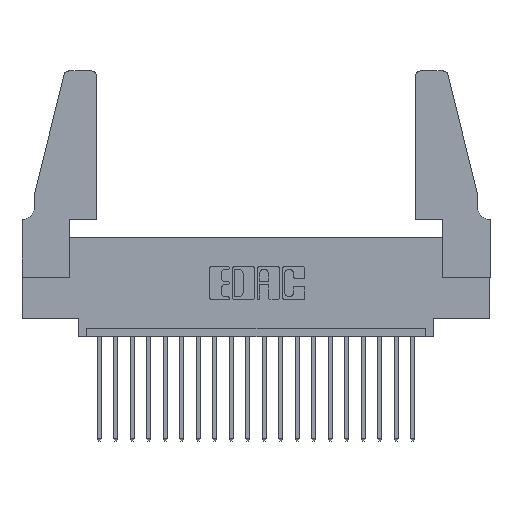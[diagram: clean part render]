
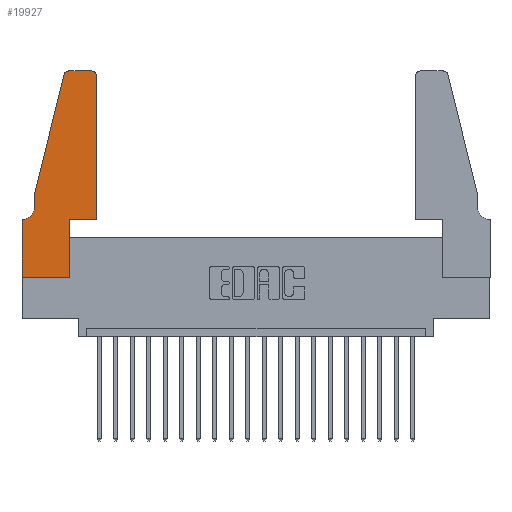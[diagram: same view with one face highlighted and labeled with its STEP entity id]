
A CAD part, top view. The second image highlights one B-rep face of the part: STEP entity #19927.
In plain terms, the highlighted planar face has unit normal (0, 0, 1).
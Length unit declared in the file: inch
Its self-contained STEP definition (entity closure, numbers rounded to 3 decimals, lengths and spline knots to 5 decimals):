
#42 = ORIENTED_EDGE ( 'NONE', *, *, #7718, .T. ) ;
#100 = EDGE_CURVE ( 'NONE', #8436, #19160, #12541, .T. ) ;
#278 = DIRECTION ( 'NONE',  ( 1., 0., 0. ) ) ;
#500 = DIRECTION ( 'NONE',  ( 1., 0., 0. ) ) ;
#636 = DIRECTION ( 'NONE',  ( 0., -1., 0. ) ) ;
#661 = CARTESIAN_POINT ( 'NONE',  ( 0.0755, 0.35, 0.37 ) ) ;
#727 = AXIS2_PLACEMENT_3D ( 'NONE', #11639, #16395, #500 ) ;
#766 = DIRECTION ( 'NONE',  ( -0.239, -0.971, 0. ) ) ;
#945 = DIRECTION ( 'NONE',  ( 0., 0., 1. ) ) ;
#1049 = DIRECTION ( 'NONE',  ( -1., 0., 0. ) ) ;
#1065 = CARTESIAN_POINT ( 'NONE',  ( 0.284, 1.25, 0.37 ) ) ;
#1090 = LINE ( 'NONE', #8948, #9182 ) ;
#1420 = CARTESIAN_POINT ( 'NONE',  ( 0., 0., 0.37 ) ) ;
#1441 = CARTESIAN_POINT ( 'NONE',  ( 0.0755, 0.5, 0.37 ) ) ;
#1651 = VERTEX_POINT ( 'NONE', #19047 ) ;
#1655 = EDGE_CURVE ( 'NONE', #8353, #12202, #19097, .T. ) ;
#1698 = FACE_OUTER_BOUND ( 'NONE', #18260, .T. ) ;
#2104 = VERTEX_POINT ( 'NONE', #13752 ) ;
#2261 = ORIENTED_EDGE ( 'NONE', *, *, #10839, .T. ) ;
#2407 = CARTESIAN_POINT ( 'NONE',  ( 0.4505, 1.22, 0.37 ) ) ;
#2546 = VERTEX_POINT ( 'NONE', #13347 ) ;
#2612 = ORIENTED_EDGE ( 'NONE', *, *, #1655, .T. ) ;
#3149 = CARTESIAN_POINT ( 'NONE',  ( 0., 0.35, 0.37 ) ) ;
#3569 = ORIENTED_EDGE ( 'NONE', *, *, #5462, .T. ) ;
#3583 = VECTOR ( 'NONE', #766, 39.37008 ) ;
#3682 = CARTESIAN_POINT ( 'NONE',  ( 0.0055, 0.35, 0.37 ) ) ;
#3754 = VERTEX_POINT ( 'NONE', #14159 ) ;
#3808 = EDGE_CURVE ( 'NONE', #2104, #8353, #8250, .T. ) ;
#3920 = VECTOR ( 'NONE', #636, 39.37008 ) ;
#4205 = CIRCLE ( 'NONE', #6808, 0.07 ) ;
#4263 = VERTEX_POINT ( 'NONE', #3682 ) ;
#4315 = DIRECTION ( 'NONE',  ( -1., 0., 0. ) ) ;
#4437 = CARTESIAN_POINT ( 'NONE',  ( 0.4505, 0.35, 0.37 ) ) ;
#4447 = DIRECTION ( 'NONE',  ( 1., 0., 0. ) ) ;
#5462 = EDGE_CURVE ( 'NONE', #19718, #19481, #8505, .T. ) ;
#6401 = LINE ( 'NONE', #661, #8649 ) ;
#6675 = CARTESIAN_POINT ( 'NONE',  ( 0., 0., 0.37 ) ) ;
#6808 = AXIS2_PLACEMENT_3D ( 'NONE', #20013, #18310, #15224 ) ;
#6945 = CARTESIAN_POINT ( 'NONE',  ( 0.0755, 0.5, 0.37 ) ) ;
#6960 = EDGE_CURVE ( 'NONE', #19160, #2546, #8687, .T. ) ;
#7383 = CARTESIAN_POINT ( 'NONE',  ( 0.4205, 1.22, 0.37 ) ) ;
#7718 = EDGE_CURVE ( 'NONE', #4263, #8436, #6401, .T. ) ;
#7729 = VERTEX_POINT ( 'NONE', #1065 ) ;
#8171 = ORIENTED_EDGE ( 'NONE', *, *, #6960, .T. ) ;
#8250 = LINE ( 'NONE', #4437, #19176 ) ;
#8353 = VERTEX_POINT ( 'NONE', #15241 ) ;
#8436 = VERTEX_POINT ( 'NONE', #15012 ) ;
#8505 = LINE ( 'NONE', #12013, #3583 ) ;
#8596 = ORIENTED_EDGE ( 'NONE', *, *, #10520, .T. ) ;
#8649 = VECTOR ( 'NONE', #4315, 39.37008 ) ;
#8687 = LINE ( 'NONE', #6675, #15054 ) ;
#8767 = ORIENTED_EDGE ( 'NONE', *, *, #19090, .T. ) ;
#8900 = ORIENTED_EDGE ( 'NONE', *, *, #3808, .T. ) ;
#8948 = CARTESIAN_POINT ( 'NONE',  ( 0.2605, 1.25, 0.37 ) ) ;
#8990 = DIRECTION ( 'NONE',  ( 1., 0., 0. ) ) ;
#9182 = VECTOR ( 'NONE', #1049, 39.37008 ) ;
#9311 = LINE ( 'NONE', #11354, #17394 ) ;
#9631 = EDGE_CURVE ( 'NONE', #19481, #3754, #16663, .T. ) ;
#9711 = DIRECTION ( 'NONE',  ( 0., 1., 0. ) ) ;
#9851 = CARTESIAN_POINT ( 'NONE',  ( 0.4505, 0.35, 0.37 ) ) ;
#10071 = EDGE_CURVE ( 'NONE', #12202, #1651, #16834, .T. ) ;
#10520 = EDGE_CURVE ( 'NONE', #1651, #7729, #1090, .T. ) ;
#10839 = EDGE_CURVE ( 'NONE', #7729, #19718, #11644, .T. ) ;
#11354 = CARTESIAN_POINT ( 'NONE',  ( 0.2865, 0.35, 0.37 ) ) ;
#11639 = CARTESIAN_POINT ( 'NONE',  ( 0.284, 1.22, 0.37 ) ) ;
#11644 = CIRCLE ( 'NONE', #727, 0.03 ) ;
#12013 = CARTESIAN_POINT ( 'NONE',  ( 0.0755, 0.5, 0.37 ) ) ;
#12202 = VERTEX_POINT ( 'NONE', #2407 ) ;
#12541 = LINE ( 'NONE', #1420, #17707 ) ;
#13213 = ORIENTED_EDGE ( 'NONE', *, *, #9631, .T. ) ;
#13347 = CARTESIAN_POINT ( 'NONE',  ( 0.2865, 0., 0.37 ) ) ;
#13750 = ORIENTED_EDGE ( 'NONE', *, *, #18132, .T. ) ;
#13752 = CARTESIAN_POINT ( 'NONE',  ( 0.2865, 0.35, 0.37 ) ) ;
#13938 = AXIS2_PLACEMENT_3D ( 'NONE', #3149, #14106, #4447 ) ;
#14106 = DIRECTION ( 'NONE',  ( 0., 0., 1. ) ) ;
#14159 = CARTESIAN_POINT ( 'NONE',  ( 0.0755, 0.42, 0.37 ) ) ;
#14477 = AXIS2_PLACEMENT_3D ( 'NONE', #7383, #945, #8990 ) ;
#15012 = CARTESIAN_POINT ( 'NONE',  ( 0., 0.35, 0.37 ) ) ;
#15054 = VECTOR ( 'NONE', #278, 39.37008 ) ;
#15224 = DIRECTION ( 'NONE',  ( -1., 0., 0. ) ) ;
#15241 = CARTESIAN_POINT ( 'NONE',  ( 0.4505, 0.35, 0.37 ) ) ;
#15765 = DIRECTION ( 'NONE',  ( 0., -1., 0. ) ) ;
#15949 = VECTOR ( 'NONE', #17682, 39.37008 ) ;
#16093 = ORIENTED_EDGE ( 'NONE', *, *, #100, .T. ) ;
#16395 = DIRECTION ( 'NONE',  ( 0., 0., 1. ) ) ;
#16663 = LINE ( 'NONE', #6945, #3920 ) ;
#16834 = CIRCLE ( 'NONE', #14477, 0.03 ) ;
#16858 = DIRECTION ( 'NONE',  ( 1., 0., 0. ) ) ;
#17193 = PLANE ( 'NONE',  #13938 ) ;
#17394 = VECTOR ( 'NONE', #9711, 39.37008 ) ;
#17682 = DIRECTION ( 'NONE',  ( 0., 1., 0. ) ) ;
#17707 = VECTOR ( 'NONE', #15765, 39.37008 ) ;
#18023 = CARTESIAN_POINT ( 'NONE',  ( 0., 0., 0.37 ) ) ;
#18132 = EDGE_CURVE ( 'NONE', #3754, #4263, #4205, .T. ) ;
#18225 = CARTESIAN_POINT ( 'NONE',  ( 0.25487, 1.22718, 0.37 ) ) ;
#18260 = EDGE_LOOP ( 'NONE', ( #8596, #2261, #3569, #13213, #13750, #42, #16093, #8171, #8767, #8900, #2612, #19181 ) ) ;
#18310 = DIRECTION ( 'NONE',  ( 0., 0., -1. ) ) ;
#19047 = CARTESIAN_POINT ( 'NONE',  ( 0.4205, 1.25, 0.37 ) ) ;
#19090 = EDGE_CURVE ( 'NONE', #2546, #2104, #9311, .T. ) ;
#19097 = LINE ( 'NONE', #9851, #15949 ) ;
#19160 = VERTEX_POINT ( 'NONE', #18023 ) ;
#19176 = VECTOR ( 'NONE', #16858, 39.37008 ) ;
#19181 = ORIENTED_EDGE ( 'NONE', *, *, #10071, .T. ) ;
#19481 = VERTEX_POINT ( 'NONE', #1441 ) ;
#19718 = VERTEX_POINT ( 'NONE', #18225 ) ;
#19927 = ADVANCED_FACE ( 'NONE', ( #1698 ), #17193, .T. ) ;
#20013 = CARTESIAN_POINT ( 'NONE',  ( 0.0055, 0.42, 0.37 ) ) ;
